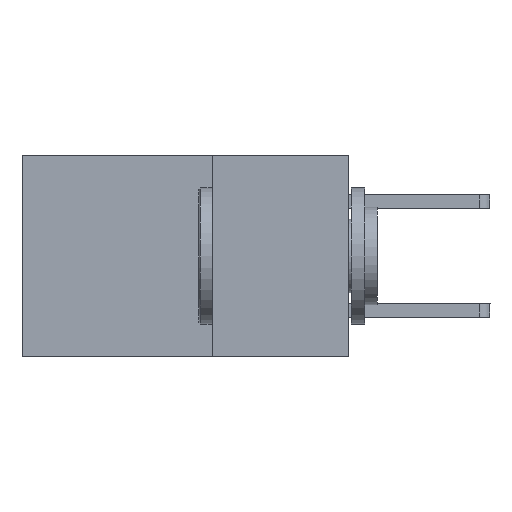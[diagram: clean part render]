
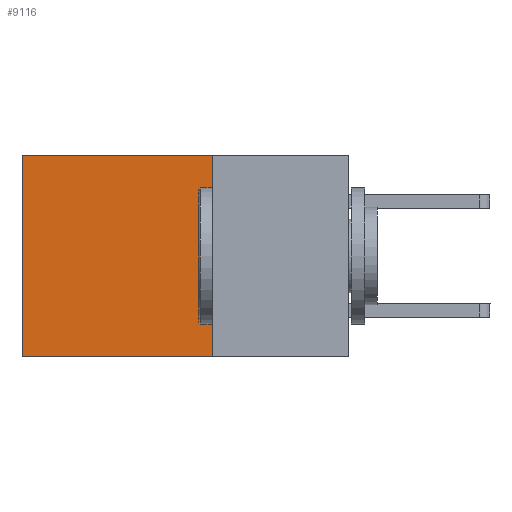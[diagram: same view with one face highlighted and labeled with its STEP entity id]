
A CAD part, left-side view. The second image highlights one B-rep face of the part: STEP entity #9116.
In plain terms, the highlighted planar face has unit normal (-1, 0, 0).
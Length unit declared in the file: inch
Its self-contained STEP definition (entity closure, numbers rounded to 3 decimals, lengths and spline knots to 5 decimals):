
#63 = CARTESIAN_POINT ( 'NONE',  ( 0.2615, 0.6, -0.37 ) ) ;
#405 = CARTESIAN_POINT ( 'NONE',  ( 0.2615, 0.6, -0.37 ) ) ;
#1083 = DIRECTION ( 'NONE',  ( 0., 0., -1. ) ) ;
#1085 = EDGE_CURVE ( 'NONE', #3474, #7164, #3327, .T. ) ;
#1123 = ORIENTED_EDGE ( 'NONE', *, *, #4531, .F. ) ;
#1233 = VECTOR ( 'NONE', #1083, 39.37008 ) ;
#1506 = CARTESIAN_POINT ( 'NONE',  ( 0.2615, 0.25, 0. ) ) ;
#1609 = PLANE ( 'NONE',  #9474 ) ;
#1680 = VECTOR ( 'NONE', #3280, 39.37008 ) ;
#1741 = EDGE_LOOP ( 'NONE', ( #7952, #1123, #7921, #1745 ) ) ;
#1745 = ORIENTED_EDGE ( 'NONE', *, *, #9044, .T. ) ;
#2402 = DIRECTION ( 'NONE',  ( 0., 0., -1. ) ) ;
#2760 = VECTOR ( 'NONE', #6205, 39.37008 ) ;
#2767 = CARTESIAN_POINT ( 'NONE',  ( 0.2615, 0.25, 0. ) ) ;
#3280 = DIRECTION ( 'NONE',  ( 0., 0., -1. ) ) ;
#3327 = LINE ( 'NONE', #405, #1233 ) ;
#3352 = CARTESIAN_POINT ( 'NONE',  ( 0.2615, 0.25, -0.37 ) ) ;
#3474 = VERTEX_POINT ( 'NONE', #9228 ) ;
#3759 = LINE ( 'NONE', #3352, #1680 ) ;
#3986 = CARTESIAN_POINT ( 'NONE',  ( 0.2615, 0.25, -0.37 ) ) ;
#4292 = FACE_OUTER_BOUND ( 'NONE', #1741, .T. ) ;
#4531 = EDGE_CURVE ( 'NONE', #6281, #7164, #7966, .T. ) ;
#5873 = DIRECTION ( 'NONE',  ( 0., 1., 0. ) ) ;
#5892 = CARTESIAN_POINT ( 'NONE',  ( 0.2615, 0.25, -0.37 ) ) ;
#6205 = DIRECTION ( 'NONE',  ( 0., 1., 0. ) ) ;
#6281 = VERTEX_POINT ( 'NONE', #3986 ) ;
#6412 = EDGE_CURVE ( 'NONE', #8749, #6281, #3759, .T. ) ;
#7119 = DIRECTION ( 'NONE',  ( 1., 0., 0. ) ) ;
#7164 = VERTEX_POINT ( 'NONE', #63 ) ;
#7921 = ORIENTED_EDGE ( 'NONE', *, *, #6412, .F. ) ;
#7952 = ORIENTED_EDGE ( 'NONE', *, *, #1085, .T. ) ;
#7966 = LINE ( 'NONE', #5892, #9774 ) ;
#8749 = VERTEX_POINT ( 'NONE', #2767 ) ;
#9038 = LINE ( 'NONE', #1506, #2760 ) ;
#9044 = EDGE_CURVE ( 'NONE', #8749, #3474, #9038, .T. ) ;
#9116 = ADVANCED_FACE ( 'NONE', ( #4292 ), #1609, .F. ) ;
#9228 = CARTESIAN_POINT ( 'NONE',  ( 0.2615, 0.6, 0. ) ) ;
#9449 = CARTESIAN_POINT ( 'NONE',  ( 0.2615, 0.25, -0.37 ) ) ;
#9474 = AXIS2_PLACEMENT_3D ( 'NONE', #9449, #7119, #2402 ) ;
#9774 = VECTOR ( 'NONE', #5873, 39.37008 ) ;
